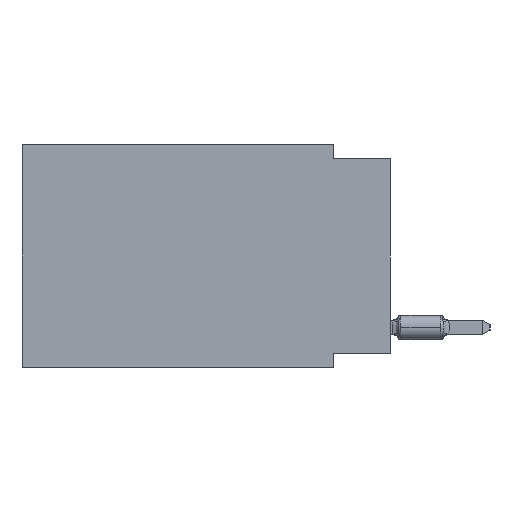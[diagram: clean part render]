
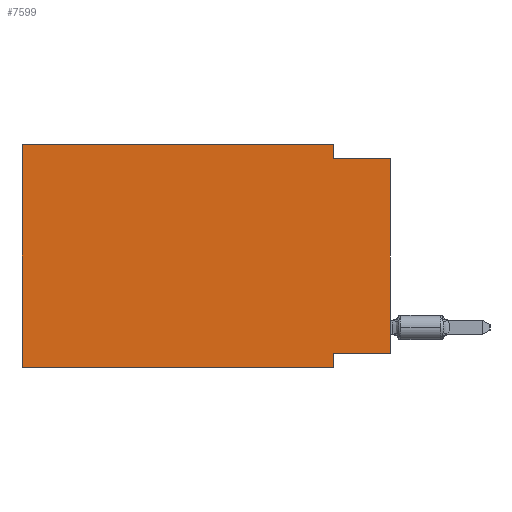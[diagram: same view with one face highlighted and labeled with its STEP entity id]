
A CAD part, left-side view. The second image highlights one B-rep face of the part: STEP entity #7599.
In plain terms, the highlighted planar face has unit normal (-1, 0, 0).
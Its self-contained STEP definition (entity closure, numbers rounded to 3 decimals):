
#252 = ORIENTED_EDGE ( 'NONE', *, *, #9950, .T. ) ;
#653 = VECTOR ( 'NONE', #34427, 1000. ) ;
#1174 = EDGE_CURVE ( 'NONE', #25967, #22125, #18269, .T. ) ;
#2514 = DIRECTION ( 'NONE',  ( 0., -1., 0. ) ) ;
#2563 = CARTESIAN_POINT ( 'NONE',  ( 0., 2.54, -0.635 ) ) ;
#2645 = VECTOR ( 'NONE', #5731, 1000. ) ;
#2696 = VECTOR ( 'NONE', #4954, 1000. ) ;
#2868 = CARTESIAN_POINT ( 'NONE',  ( 0., 0., -0.635 ) ) ;
#3070 = LINE ( 'NONE', #6037, #6394 ) ;
#3426 = VERTEX_POINT ( 'NONE', #34549 ) ;
#3878 = DIRECTION ( 'NONE',  ( 0., 0., -1. ) ) ;
#4954 = DIRECTION ( 'NONE',  ( 0., 0., 1. ) ) ;
#4967 = EDGE_CURVE ( 'NONE', #12165, #30015, #32396, .T. ) ;
#5133 = ORIENTED_EDGE ( 'NONE', *, *, #8887, .F. ) ;
#5318 = LINE ( 'NONE', #10761, #21239 ) ;
#5429 = ORIENTED_EDGE ( 'NONE', *, *, #1174, .F. ) ;
#5575 = VERTEX_POINT ( 'NONE', #2563 ) ;
#5642 = CARTESIAN_POINT ( 'NONE',  ( 0., 16.383, -9.906 ) ) ;
#5731 = DIRECTION ( 'NONE',  ( 0., 0., -1. ) ) ;
#6037 = CARTESIAN_POINT ( 'NONE',  ( 0., 0., 0. ) ) ;
#6394 = VECTOR ( 'NONE', #21636, 1000. ) ;
#6571 = EDGE_CURVE ( 'NONE', #28333, #3426, #3070, .T. ) ;
#6638 = VECTOR ( 'NONE', #29508, 1000. ) ;
#7599 = ADVANCED_FACE ( 'NONE', ( #33188 ), #25603, .F. ) ;
#8309 = DIRECTION ( 'NONE',  ( 0., 1., 0. ) ) ;
#8340 = CARTESIAN_POINT ( 'NONE',  ( 0., 2.54, -9.906 ) ) ;
#8789 = ORIENTED_EDGE ( 'NONE', *, *, #20127, .F. ) ;
#8887 = EDGE_CURVE ( 'NONE', #28333, #12165, #34653, .T. ) ;
#9950 = EDGE_CURVE ( 'NONE', #25967, #30015, #18959, .T. ) ;
#10043 = CARTESIAN_POINT ( 'NONE',  ( 0., 16.383, 0. ) ) ;
#10295 = CARTESIAN_POINT ( 'NONE',  ( 0., 2.54, -9.906 ) ) ;
#10706 = CARTESIAN_POINT ( 'NONE',  ( 0., 16.383, 0. ) ) ;
#10761 = CARTESIAN_POINT ( 'NONE',  ( 0., 16.383, 0. ) ) ;
#11446 = CARTESIAN_POINT ( 'NONE',  ( 0., 16.383, -9.906 ) ) ;
#12103 = CARTESIAN_POINT ( 'NONE',  ( 0., 2.54, -9.271 ) ) ;
#12165 = VERTEX_POINT ( 'NONE', #12103 ) ;
#17135 = ORIENTED_EDGE ( 'NONE', *, *, #6571, .T. ) ;
#18070 = DIRECTION ( 'NONE',  ( 0., 0., -1. ) ) ;
#18241 = CARTESIAN_POINT ( 'NONE',  ( 0., 2.54, 0. ) ) ;
#18269 = LINE ( 'NONE', #10043, #2696 ) ;
#18803 = LINE ( 'NONE', #2868, #6638 ) ;
#18959 = LINE ( 'NONE', #5642, #653 ) ;
#18979 = EDGE_CURVE ( 'NONE', #5575, #3426, #18803, .T. ) ;
#19651 = CARTESIAN_POINT ( 'NONE',  ( 0., 0., -9.271 ) ) ;
#19661 = CARTESIAN_POINT ( 'NONE',  ( 0., 16.383, 0. ) ) ;
#20127 = EDGE_CURVE ( 'NONE', #22125, #25832, #5318, .T. ) ;
#20859 = ORIENTED_EDGE ( 'NONE', *, *, #26897, .F. ) ;
#21239 = VECTOR ( 'NONE', #2514, 1000. ) ;
#21437 = CARTESIAN_POINT ( 'NONE',  ( 0., 2.54, 0. ) ) ;
#21562 = ORIENTED_EDGE ( 'NONE', *, *, #4967, .F. ) ;
#21636 = DIRECTION ( 'NONE',  ( 0., 0., 1. ) ) ;
#22125 = VERTEX_POINT ( 'NONE', #10706 ) ;
#22976 = VECTOR ( 'NONE', #18070, 1000. ) ;
#23332 = LINE ( 'NONE', #18241, #22976 ) ;
#24173 = EDGE_LOOP ( 'NONE', ( #17135, #33332, #20859, #8789, #5429, #252, #21562, #5133 ) ) ;
#25603 = PLANE ( 'NONE',  #32460 ) ;
#25832 = VERTEX_POINT ( 'NONE', #21437 ) ;
#25967 = VERTEX_POINT ( 'NONE', #11446 ) ;
#26897 = EDGE_CURVE ( 'NONE', #25832, #5575, #23332, .T. ) ;
#26925 = CARTESIAN_POINT ( 'NONE',  ( 0., 0., -9.271 ) ) ;
#28333 = VERTEX_POINT ( 'NONE', #19651 ) ;
#29508 = DIRECTION ( 'NONE',  ( 0., -1., 0. ) ) ;
#30015 = VERTEX_POINT ( 'NONE', #10295 ) ;
#31372 = VECTOR ( 'NONE', #8309, 1000. ) ;
#32396 = LINE ( 'NONE', #8340, #2645 ) ;
#32460 = AXIS2_PLACEMENT_3D ( 'NONE', #19661, #33695, #3878 ) ;
#33188 = FACE_OUTER_BOUND ( 'NONE', #24173, .T. ) ;
#33332 = ORIENTED_EDGE ( 'NONE', *, *, #18979, .F. ) ;
#33695 = DIRECTION ( 'NONE',  ( 1., 0., 0. ) ) ;
#34427 = DIRECTION ( 'NONE',  ( 0., -1., 0. ) ) ;
#34549 = CARTESIAN_POINT ( 'NONE',  ( 0., 0., -0.635 ) ) ;
#34653 = LINE ( 'NONE', #26925, #31372 ) ;
